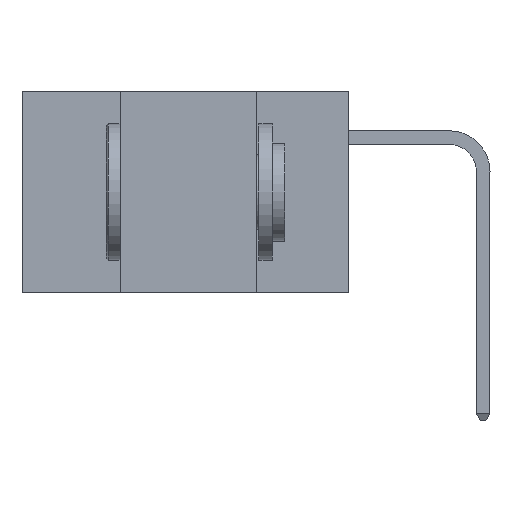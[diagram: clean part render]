
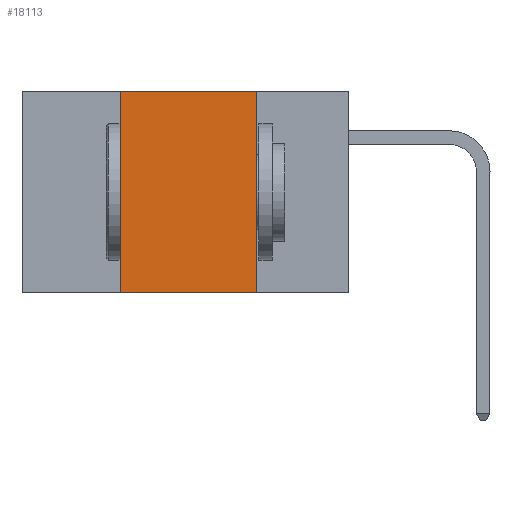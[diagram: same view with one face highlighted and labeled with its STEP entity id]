
A CAD part, left-side view. The second image highlights one B-rep face of the part: STEP entity #18113.
In plain terms, the highlighted planar face has unit normal (-1, 0, 0).
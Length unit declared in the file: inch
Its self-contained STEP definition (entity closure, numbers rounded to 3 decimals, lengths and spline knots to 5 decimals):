
#9 = VECTOR ( 'NONE', #19260, 39.37008 ) ;
#118 = EDGE_CURVE ( 'NONE', #13190, #8420, #4506, .T. ) ;
#721 = CARTESIAN_POINT ( 'NONE',  ( 0., 0.6, 0. ) ) ;
#847 = EDGE_CURVE ( 'NONE', #6061, #8420, #5550, .T. ) ;
#2276 = AXIS2_PLACEMENT_3D ( 'NONE', #6755, #8569, #10233 ) ;
#2374 = ORIENTED_EDGE ( 'NONE', *, *, #7256, .F. ) ;
#2491 = DIRECTION ( 'NONE',  ( 0., -1., 0. ) ) ;
#2829 = VERTEX_POINT ( 'NONE', #20575 ) ;
#3070 = LINE ( 'NONE', #4539, #5287 ) ;
#3179 = PLANE ( 'NONE',  #2276 ) ;
#4215 = CARTESIAN_POINT ( 'NONE',  ( 0., 0.6, -0.37 ) ) ;
#4506 = LINE ( 'NONE', #4215, #14860 ) ;
#4539 = CARTESIAN_POINT ( 'NONE',  ( 0., 0.42, 0. ) ) ;
#5224 = LINE ( 'NONE', #721, #21745 ) ;
#5287 = VECTOR ( 'NONE', #6335, 39.37008 ) ;
#5550 = LINE ( 'NONE', #20830, #9 ) ;
#6061 = VERTEX_POINT ( 'NONE', #10968 ) ;
#6335 = DIRECTION ( 'NONE',  ( 0., 0., 1. ) ) ;
#6755 = CARTESIAN_POINT ( 'NONE',  ( 0., 0.6, 0. ) ) ;
#7256 = EDGE_CURVE ( 'NONE', #13190, #2829, #3070, .T. ) ;
#8378 = EDGE_CURVE ( 'NONE', #2829, #6061, #5224, .T. ) ;
#8420 = VERTEX_POINT ( 'NONE', #20775 ) ;
#8569 = DIRECTION ( 'NONE',  ( 1., 0., 0. ) ) ;
#10233 = DIRECTION ( 'NONE',  ( 0., 0., -1. ) ) ;
#10968 = CARTESIAN_POINT ( 'NONE',  ( 0., 0.17, 0. ) ) ;
#13190 = VERTEX_POINT ( 'NONE', #16479 ) ;
#13247 = DIRECTION ( 'NONE',  ( 0., -1., 0. ) ) ;
#14773 = EDGE_LOOP ( 'NONE', ( #17695, #22398, #2374, #17733 ) ) ;
#14860 = VECTOR ( 'NONE', #2491, 39.37008 ) ;
#16479 = CARTESIAN_POINT ( 'NONE',  ( 0., 0.42, -0.37 ) ) ;
#17695 = ORIENTED_EDGE ( 'NONE', *, *, #847, .F. ) ;
#17733 = ORIENTED_EDGE ( 'NONE', *, *, #118, .T. ) ;
#18113 = ADVANCED_FACE ( 'NONE', ( #19821 ), #3179, .F. ) ;
#19260 = DIRECTION ( 'NONE',  ( 0., 0., -1. ) ) ;
#19821 = FACE_OUTER_BOUND ( 'NONE', #14773, .T. ) ;
#20575 = CARTESIAN_POINT ( 'NONE',  ( 0., 0.42, 0. ) ) ;
#20775 = CARTESIAN_POINT ( 'NONE',  ( 0., 0.17, -0.37 ) ) ;
#20830 = CARTESIAN_POINT ( 'NONE',  ( 0., 0.17, 0. ) ) ;
#21745 = VECTOR ( 'NONE', #13247, 39.37008 ) ;
#22398 = ORIENTED_EDGE ( 'NONE', *, *, #8378, .F. ) ;
